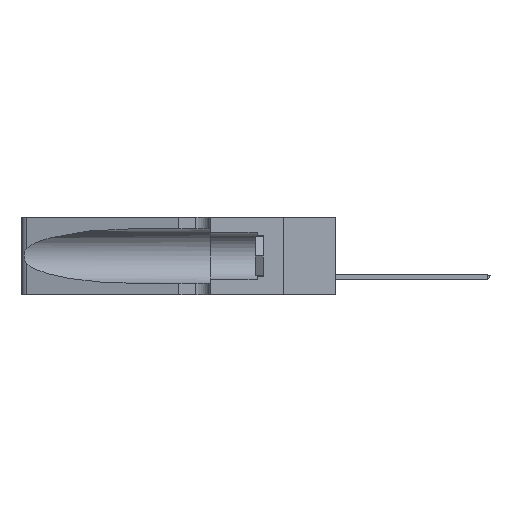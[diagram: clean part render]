
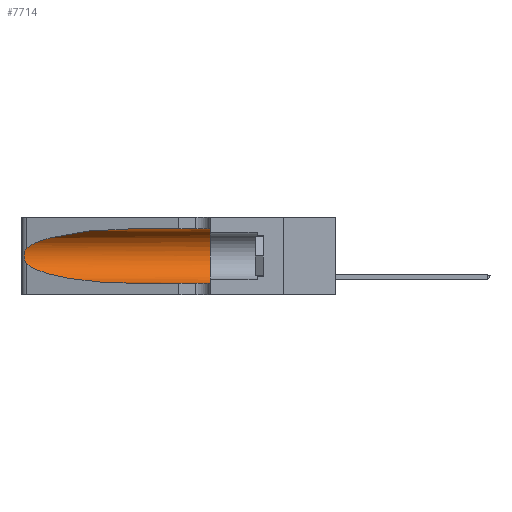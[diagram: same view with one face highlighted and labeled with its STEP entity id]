
A CAD part, left-side view. The second image highlights one B-rep face of the part: STEP entity #7714.
In plain terms, the highlighted cylindrical face has radius 3.308 mm (diameter 6.617 mm), a partial arc.
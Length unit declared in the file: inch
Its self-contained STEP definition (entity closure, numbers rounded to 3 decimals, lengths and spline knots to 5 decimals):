
#1179 = CARTESIAN_POINT ( 'NONE',  ( 0.1305, 1.61858, 0.31525 ) ) ;
#1200 = CARTESIAN_POINT ( 'NONE',  ( 0.25487, 1.22718, 0.22369 ) ) ;
#1726 = CARTESIAN_POINT ( 'NONE',  ( 0.1305, 1.61858, 0.185 ) ) ;
#2959 = CARTESIAN_POINT ( 'NONE',  ( 0.25487, 1.22718, 0.14631 ) ) ;
#3447 = FACE_OUTER_BOUND ( 'NONE', #24798, .T. ) ;
#4015 = CARTESIAN_POINT ( 'NONE',  ( 0.1305, 0.72297, 0.05475 ) ) ;
#4985 = CARTESIAN_POINT ( 'NONE',  ( 0.25787, 1.23484, 0.2124 ) ) ;
#5333 = CARTESIAN_POINT ( 'NONE',  ( 0.25639, 1.23186, 0.15144 ) ) ;
#5608 = CARTESIAN_POINT ( 'NONE',  ( 0.2373, 1.15595, 0.28018 ) ) ;
#6973 = VERTEX_POINT ( 'NONE', #43331 ) ;
#7714 = ADVANCED_FACE ( 'NONE', ( #3447 ), #45612, .F. ) ;
#8480 = CARTESIAN_POINT ( 'NONE',  ( 0.25639, 1.23184, 0.21858 ) ) ;
#8800 = CARTESIAN_POINT ( 'NONE',  ( 0.26075, 1.23896, 0.19203 ) ) ;
#10278 = VERTEX_POINT ( 'NONE', #21001 ) ;
#10604 = VERTEX_POINT ( 'NONE', #4015 ) ;
#12086 = CARTESIAN_POINT ( 'NONE',  ( 0.1305, 1.61858, 0.05475 ) ) ;
#12254 =( BOUNDED_CURVE ( )  B_SPLINE_CURVE ( 3, ( #41307, #15974, #5608, #19760 ),
 .UNSPECIFIED., .F., .F. ) 
 B_SPLINE_CURVE_WITH_KNOTS ( ( 4, 4 ),
 ( 1.5708, 2.84003 ),
 .UNSPECIFIED. ) 
 CURVE ( )  GEOMETRIC_REPRESENTATION_ITEM ( )  RATIONAL_B_SPLINE_CURVE ( ( 1., 0.87, 0.87, 1. ) ) 
 REPRESENTATION_ITEM ( '' )  );
#13357 = CARTESIAN_POINT ( 'NONE',  ( 0.1305, 0.72297, 0.05475 ) ) ;
#14923 = VERTEX_POINT ( 'NONE', #38186 ) ;
#15974 = CARTESIAN_POINT ( 'NONE',  ( 0.18966, 0.96281, 0.31525 ) ) ;
#17067 = DIRECTION ( 'NONE',  ( 0., -1., 0. ) ) ;
#17526 = EDGE_CURVE ( 'NONE', #31070, #6973, #43655, .T. ) ;
#19760 = CARTESIAN_POINT ( 'NONE',  ( 0.25487, 1.22718, 0.22369 ) ) ;
#19985 = CARTESIAN_POINT ( 'NONE',  ( 0.26018, 1.23835, 0.19895 ) ) ;
#20396 = DIRECTION ( 'NONE',  ( 0., 0., -1. ) ) ;
#20412 = CARTESIAN_POINT ( 'NONE',  ( 0.1305, 0.35, 0.05475 ) ) ;
#21001 = CARTESIAN_POINT ( 'NONE',  ( 0.25487, 1.22718, 0.14631 ) ) ;
#21903 = CARTESIAN_POINT ( 'NONE',  ( 0.1305, 0.72297, 0.31525 ) ) ;
#21930 = CIRCLE ( 'NONE', #28462, 0.13025 ) ;
#22789 = CARTESIAN_POINT ( 'NONE',  ( 0.1305, 0.35, 0.185 ) ) ;
#23139 = CARTESIAN_POINT ( 'NONE',  ( 0.26017, 1.23833, 0.17102 ) ) ;
#23173 = ORIENTED_EDGE ( 'NONE', *, *, #23476, .T. ) ;
#23476 = EDGE_CURVE ( 'NONE', #10604, #35691, #34542, .T. ) ;
#23754 = DIRECTION ( 'NONE',  ( 0., 0., 1. ) ) ;
#24630 = EDGE_CURVE ( 'NONE', #6973, #35691, #21930, .T. ) ;
#24798 = EDGE_LOOP ( 'NONE', ( #39449, #25847, #42486, #23173, #42859, #33390 ) ) ;
#25837 = EDGE_CURVE ( 'NONE', #10278, #10604, #39709, .T. ) ;
#25847 = ORIENTED_EDGE ( 'NONE', *, *, #42991, .T. ) ;
#27205 = DIRECTION ( 'NONE',  ( 0., 1., 0. ) ) ;
#28462 = AXIS2_PLACEMENT_3D ( 'NONE', #22789, #27205, #23754 ) ;
#30507 = CARTESIAN_POINT ( 'NONE',  ( 0.25555, 1.22993, 0.14849 ) ) ;
#30671 = CARTESIAN_POINT ( 'NONE',  ( 0.25854, 1.2359, 0.20912 ) ) ;
#31024 = CARTESIAN_POINT ( 'NONE',  ( 0.25789, 1.23486, 0.15765 ) ) ;
#31025 = EDGE_CURVE ( 'NONE', #31070, #14923, #12254, .T. ) ;
#31070 = VERTEX_POINT ( 'NONE', #21903 ) ;
#31911 = AXIS2_PLACEMENT_3D ( 'NONE', #1726, #34740, #20396 ) ;
#33390 = ORIENTED_EDGE ( 'NONE', *, *, #17526, .F. ) ;
#34322 = CARTESIAN_POINT ( 'NONE',  ( 0.25856, 1.23593, 0.16098 ) ) ;
#34542 = LINE ( 'NONE', #12086, #42405 ) ;
#34740 = DIRECTION ( 'NONE',  ( 0., -1., 0. ) ) ;
#34936 = CARTESIAN_POINT ( 'NONE',  ( 0.18966, 0.96281, 0.05475 ) ) ;
#35691 = VERTEX_POINT ( 'NONE', #20412 ) ;
#36960 = CARTESIAN_POINT ( 'NONE',  ( 0.25555, 1.22994, 0.2215 ) ) ;
#38186 = CARTESIAN_POINT ( 'NONE',  ( 0.25487, 1.22718, 0.22369 ) ) ;
#39449 = ORIENTED_EDGE ( 'NONE', *, *, #31025, .T. ) ;
#39709 =( BOUNDED_CURVE ( )  B_SPLINE_CURVE ( 3, ( #2959, #46208, #34936, #13357 ),
 .UNSPECIFIED., .F., .T. ) 
 B_SPLINE_CURVE_WITH_KNOTS ( ( 4, 4 ),
 ( 3.44316, 4.71239 ),
 .UNSPECIFIED. ) 
 CURVE ( )  GEOMETRIC_REPRESENTATION_ITEM ( )  RATIONAL_B_SPLINE_CURVE ( ( 1., 0.87, 0.87, 1. ) ) 
 REPRESENTATION_ITEM ( '' )  );
#40230 = B_SPLINE_CURVE_WITH_KNOTS ( 'NONE', 3,
 ( #1200, #36960, #8480, #4985, #30671, #19985, #8800, #45143, #23139, #34322, #31024, #5333, #30507, #41373 ),
 .UNSPECIFIED., .F., .F.,
 ( 4, 2, 2, 2, 2, 2, 4 ),
 ( 0., 0.00027, 0.00053, 0.00107, 0.0016, 0.00187, 0.00214 ),
 .UNSPECIFIED. ) ;
#40731 = DIRECTION ( 'NONE',  ( 0., -1., 0. ) ) ;
#41307 = CARTESIAN_POINT ( 'NONE',  ( 0.1305, 0.72297, 0.31525 ) ) ;
#41373 = CARTESIAN_POINT ( 'NONE',  ( 0.25487, 1.22718, 0.14631 ) ) ;
#42405 = VECTOR ( 'NONE', #40731, 39.37008 ) ;
#42486 = ORIENTED_EDGE ( 'NONE', *, *, #25837, .T. ) ;
#42622 = VECTOR ( 'NONE', #17067, 39.37008 ) ;
#42859 = ORIENTED_EDGE ( 'NONE', *, *, #24630, .F. ) ;
#42991 = EDGE_CURVE ( 'NONE', #14923, #10278, #40230, .T. ) ;
#43331 = CARTESIAN_POINT ( 'NONE',  ( 0.1305, 0.35, 0.31525 ) ) ;
#43655 = LINE ( 'NONE', #1179, #42622 ) ;
#45143 = CARTESIAN_POINT ( 'NONE',  ( 0.26075, 1.23896, 0.178 ) ) ;
#45612 = CYLINDRICAL_SURFACE ( 'NONE', #31911, 0.13025 ) ;
#46208 = CARTESIAN_POINT ( 'NONE',  ( 0.2373, 1.15595, 0.08982 ) ) ;
